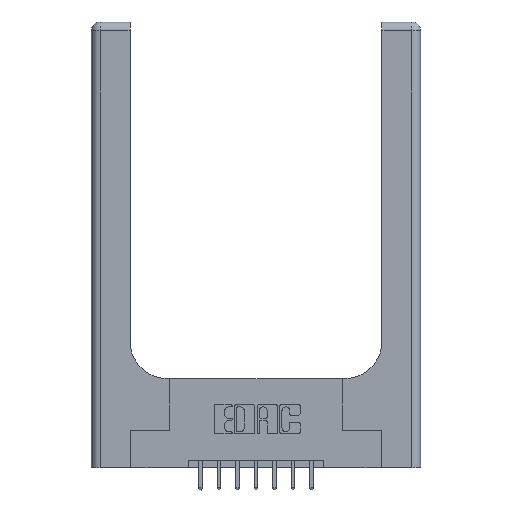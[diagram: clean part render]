
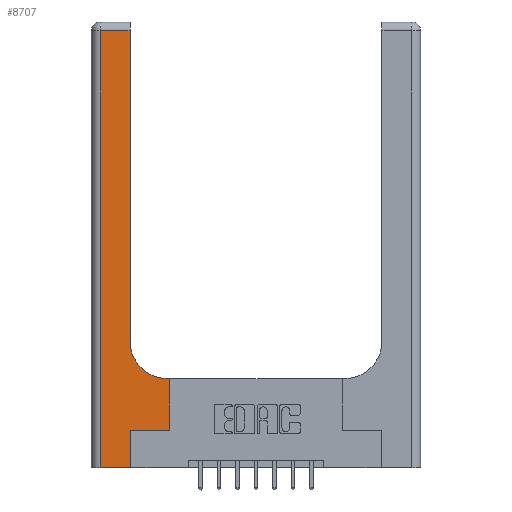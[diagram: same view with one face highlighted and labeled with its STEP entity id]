
A CAD part, top view. The second image highlights one B-rep face of the part: STEP entity #8707.
In plain terms, the highlighted planar face has unit normal (0, 0, 1).
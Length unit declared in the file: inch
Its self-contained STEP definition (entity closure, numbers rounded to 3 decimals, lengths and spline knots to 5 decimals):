
#206 = LINE ( 'NONE', #1538, #10699 ) ;
#356 = VERTEX_POINT ( 'NONE', #13667 ) ;
#376 = EDGE_LOOP ( 'NONE', ( #13248, #5936, #7373, #7501, #557, #11512, #9456, #4928, #9523 ) ) ;
#458 = CARTESIAN_POINT ( 'NONE',  ( 0.26, 0.85, 0.37 ) ) ;
#557 = ORIENTED_EDGE ( 'NONE', *, *, #5468, .T. ) ;
#696 = DIRECTION ( 'NONE',  ( 0., -1., 0. ) ) ;
#1013 = VECTOR ( 'NONE', #11205, 39.37008 ) ;
#1122 = CARTESIAN_POINT ( 'NONE',  ( 0.06, 2.94, 0.37 ) ) ;
#1130 = DIRECTION ( 'NONE',  ( 0., 0., -1. ) ) ;
#1538 = CARTESIAN_POINT ( 'NONE',  ( 0., 2.94, 0.37 ) ) ;
#1608 = VECTOR ( 'NONE', #7163, 39.37008 ) ;
#2252 = DIRECTION ( 'NONE',  ( 1., 0., 0. ) ) ;
#2281 = VERTEX_POINT ( 'NONE', #10497 ) ;
#2384 = CARTESIAN_POINT ( 'NONE',  ( 0.265, 0., 0.37 ) ) ;
#2598 = DIRECTION ( 'NONE',  ( -1., 0., 0. ) ) ;
#3286 = LINE ( 'NONE', #13549, #1013 ) ;
#3399 = EDGE_CURVE ( 'NONE', #7692, #12292, #206, .T. ) ;
#3634 = AXIS2_PLACEMENT_3D ( 'NONE', #7043, #6894, #12503 ) ;
#3661 = DIRECTION ( 'NONE',  ( 0., 1., 0. ) ) ;
#3705 = VECTOR ( 'NONE', #13860, 39.37008 ) ;
#3909 = EDGE_CURVE ( 'NONE', #12292, #10167, #12264, .T. ) ;
#4173 = LINE ( 'NONE', #12959, #13670 ) ;
#4263 = EDGE_CURVE ( 'NONE', #6123, #4539, #4173, .T. ) ;
#4539 = VERTEX_POINT ( 'NONE', #11439 ) ;
#4928 = ORIENTED_EDGE ( 'NONE', *, *, #8851, .T. ) ;
#4978 = DIRECTION ( 'NONE',  ( -1., 0., 0. ) ) ;
#5327 = EDGE_CURVE ( 'NONE', #2281, #6123, #3286, .T. ) ;
#5468 = EDGE_CURVE ( 'NONE', #13454, #2281, #9948, .T. ) ;
#5568 = VERTEX_POINT ( 'NONE', #458 ) ;
#5936 = ORIENTED_EDGE ( 'NONE', *, *, #3399, .T. ) ;
#6123 = VERTEX_POINT ( 'NONE', #13524 ) ;
#6369 = CARTESIAN_POINT ( 'NONE',  ( 0.06, 3., 0.37 ) ) ;
#6643 = VECTOR ( 'NONE', #2252, 39.37008 ) ;
#6894 = DIRECTION ( 'NONE',  ( 0., 0., -1. ) ) ;
#7043 = CARTESIAN_POINT ( 'NONE',  ( 0.51, 0.85, 0.37 ) ) ;
#7163 = DIRECTION ( 'NONE',  ( -1., 0., 0. ) ) ;
#7373 = ORIENTED_EDGE ( 'NONE', *, *, #3909, .T. ) ;
#7377 = VECTOR ( 'NONE', #696, 39.37008 ) ;
#7501 = ORIENTED_EDGE ( 'NONE', *, *, #11799, .T. ) ;
#7692 = VERTEX_POINT ( 'NONE', #13175 ) ;
#7734 = CARTESIAN_POINT ( 'NONE',  ( 0., 0., 0.37 ) ) ;
#8035 = PLANE ( 'NONE',  #8207 ) ;
#8145 = CARTESIAN_POINT ( 'NONE',  ( 0.265, 0., 0.37 ) ) ;
#8207 = AXIS2_PLACEMENT_3D ( 'NONE', #9169, #1130, #2598 ) ;
#8392 = CARTESIAN_POINT ( 'NONE',  ( 0.06, 0., 0.37 ) ) ;
#8408 = DIRECTION ( 'NONE',  ( 0., 1., 0. ) ) ;
#8499 = CIRCLE ( 'NONE', #3634, 0.25 ) ;
#8707 = ADVANCED_FACE ( 'NONE', ( #13881 ), #8035, .F. ) ;
#8829 = EDGE_CURVE ( 'NONE', #5568, #7692, #13551, .T. ) ;
#8851 = EDGE_CURVE ( 'NONE', #4539, #356, #10549, .T. ) ;
#9169 = CARTESIAN_POINT ( 'NONE',  ( 0., 3., 0.37 ) ) ;
#9456 = ORIENTED_EDGE ( 'NONE', *, *, #4263, .T. ) ;
#9523 = ORIENTED_EDGE ( 'NONE', *, *, #14427, .T. ) ;
#9948 = LINE ( 'NONE', #8145, #12948 ) ;
#10167 = VERTEX_POINT ( 'NONE', #8392 ) ;
#10497 = CARTESIAN_POINT ( 'NONE',  ( 0.265, 0.25, 0.37 ) ) ;
#10502 = LINE ( 'NONE', #7734, #6643 ) ;
#10549 = LINE ( 'NONE', #12669, #1608 ) ;
#10699 = VECTOR ( 'NONE', #4978, 39.37008 ) ;
#11205 = DIRECTION ( 'NONE',  ( 1., 0., 0. ) ) ;
#11439 = CARTESIAN_POINT ( 'NONE',  ( 0.528, 0.6, 0.37 ) ) ;
#11512 = ORIENTED_EDGE ( 'NONE', *, *, #5327, .T. ) ;
#11799 = EDGE_CURVE ( 'NONE', #10167, #13454, #10502, .T. ) ;
#12264 = LINE ( 'NONE', #6369, #7377 ) ;
#12292 = VERTEX_POINT ( 'NONE', #1122 ) ;
#12503 = DIRECTION ( 'NONE',  ( 1., 0., 0. ) ) ;
#12669 = CARTESIAN_POINT ( 'NONE',  ( 0.26, 0.6, 0.37 ) ) ;
#12768 = CARTESIAN_POINT ( 'NONE',  ( 0.26, 3., 0.37 ) ) ;
#12948 = VECTOR ( 'NONE', #3661, 39.37008 ) ;
#12959 = CARTESIAN_POINT ( 'NONE',  ( 0.528, 0.25, 0.37 ) ) ;
#13175 = CARTESIAN_POINT ( 'NONE',  ( 0.26, 2.94, 0.37 ) ) ;
#13248 = ORIENTED_EDGE ( 'NONE', *, *, #8829, .T. ) ;
#13454 = VERTEX_POINT ( 'NONE', #2384 ) ;
#13524 = CARTESIAN_POINT ( 'NONE',  ( 0.528, 0.25, 0.37 ) ) ;
#13549 = CARTESIAN_POINT ( 'NONE',  ( 0.265, 0.25, 0.37 ) ) ;
#13551 = LINE ( 'NONE', #12768, #3705 ) ;
#13667 = CARTESIAN_POINT ( 'NONE',  ( 0.51, 0.6, 0.37 ) ) ;
#13670 = VECTOR ( 'NONE', #8408, 39.37008 ) ;
#13860 = DIRECTION ( 'NONE',  ( 0., 1., 0. ) ) ;
#13881 = FACE_OUTER_BOUND ( 'NONE', #376, .T. ) ;
#14427 = EDGE_CURVE ( 'NONE', #356, #5568, #8499, .T. ) ;
